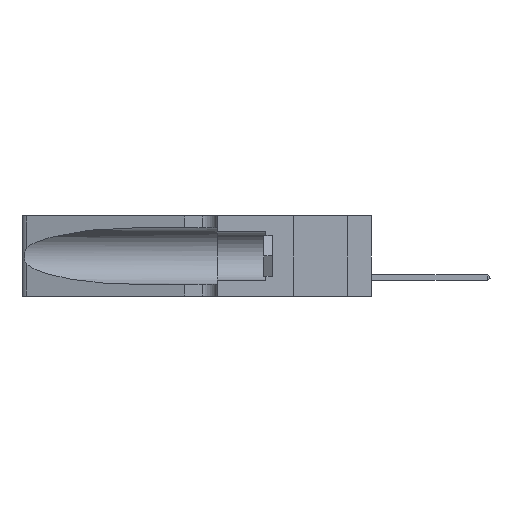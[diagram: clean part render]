
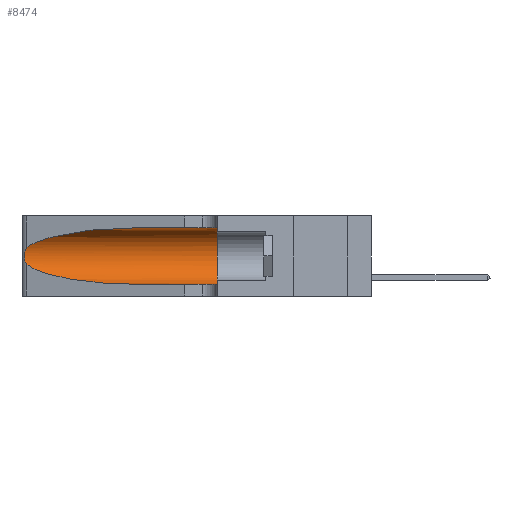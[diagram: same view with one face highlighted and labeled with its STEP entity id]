
A CAD part, left-side view. The second image highlights one B-rep face of the part: STEP entity #8474.
In plain terms, the highlighted cylindrical face has radius 3.308 mm (diameter 6.617 mm), a partial arc.
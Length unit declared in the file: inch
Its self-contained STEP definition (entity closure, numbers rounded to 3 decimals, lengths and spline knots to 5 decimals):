
#610 = VERTEX_POINT ( 'NONE', #5513 ) ;
#1059 = CARTESIAN_POINT ( 'NONE',  ( 0.25639, 1.23184, 0.21858 ) ) ;
#1222 = DIRECTION ( 'NONE',  ( 0., -1., 0. ) ) ;
#1430 = FACE_OUTER_BOUND ( 'NONE', #3080, .T. ) ;
#1438 =( BOUNDED_CURVE ( )  B_SPLINE_CURVE ( 3, ( #1781, #30792, #2269, #8991 ),
 .UNSPECIFIED., .F., .F. ) 
 B_SPLINE_CURVE_WITH_KNOTS ( ( 4, 4 ),
 ( 1.5708, 2.84003 ),
 .UNSPECIFIED. ) 
 CURVE ( )  GEOMETRIC_REPRESENTATION_ITEM ( )  RATIONAL_B_SPLINE_CURVE ( ( 1., 0.87, 0.87, 1. ) ) 
 REPRESENTATION_ITEM ( '' )  );
#1781 = CARTESIAN_POINT ( 'NONE',  ( 0.1305, 0.72297, 0.31525 ) ) ;
#1903 = CARTESIAN_POINT ( 'NONE',  ( 0.2373, 1.15595, 0.08982 ) ) ;
#2073 = CARTESIAN_POINT ( 'NONE',  ( 0.1305, 0.72297, 0.05475 ) ) ;
#2269 = CARTESIAN_POINT ( 'NONE',  ( 0.2373, 1.15595, 0.28018 ) ) ;
#2983 = CARTESIAN_POINT ( 'NONE',  ( 0.25789, 1.23486, 0.15765 ) ) ;
#3080 = EDGE_LOOP ( 'NONE', ( #33005, #5536, #32634, #36793, #13615, #35650 ) ) ;
#3566 = VERTEX_POINT ( 'NONE', #28455 ) ;
#5513 = CARTESIAN_POINT ( 'NONE',  ( 0.1305, 0.35, 0.05475 ) ) ;
#5536 = ORIENTED_EDGE ( 'NONE', *, *, #34141, .T. ) ;
#5541 = VECTOR ( 'NONE', #1222, 39.37008 ) ;
#5923 = CARTESIAN_POINT ( 'NONE',  ( 0.25787, 1.23484, 0.2124 ) ) ;
#6444 = DIRECTION ( 'NONE',  ( 0., 0., -1. ) ) ;
#7768 = CARTESIAN_POINT ( 'NONE',  ( 0.25856, 1.23593, 0.16098 ) ) ;
#8166 = CYLINDRICAL_SURFACE ( 'NONE', #24331, 0.13025 ) ;
#8474 = ADVANCED_FACE ( 'NONE', ( #1430 ), #8166, .F. ) ;
#8942 = EDGE_CURVE ( 'NONE', #27003, #3566, #13263, .T. ) ;
#8991 = CARTESIAN_POINT ( 'NONE',  ( 0.25487, 1.22718, 0.22369 ) ) ;
#10820 = EDGE_CURVE ( 'NONE', #31701, #45559, #1438, .T. ) ;
#13191 = CARTESIAN_POINT ( 'NONE',  ( 0.26075, 1.23896, 0.178 ) ) ;
#13263 =( BOUNDED_CURVE ( )  B_SPLINE_CURVE ( 3, ( #30753, #1903, #41565, #2073 ),
 .UNSPECIFIED., .F., .F. ) 
 B_SPLINE_CURVE_WITH_KNOTS ( ( 4, 4 ),
 ( 3.44316, 4.71239 ),
 .UNSPECIFIED. ) 
 CURVE ( )  GEOMETRIC_REPRESENTATION_ITEM ( )  RATIONAL_B_SPLINE_CURVE ( ( 1., 0.87, 0.87, 1. ) ) 
 REPRESENTATION_ITEM ( '' )  );
#13466 = EDGE_CURVE ( 'NONE', #35934, #610, #22303, .T. ) ;
#13615 = ORIENTED_EDGE ( 'NONE', *, *, #13466, .F. ) ;
#15055 = CARTESIAN_POINT ( 'NONE',  ( 0.25487, 1.22718, 0.14631 ) ) ;
#15162 = CARTESIAN_POINT ( 'NONE',  ( 0.25487, 1.22718, 0.22369 ) ) ;
#15332 = CARTESIAN_POINT ( 'NONE',  ( 0.1305, 1.61858, 0.31525 ) ) ;
#16100 = CARTESIAN_POINT ( 'NONE',  ( 0.26018, 1.23835, 0.19895 ) ) ;
#16700 = B_SPLINE_CURVE_WITH_KNOTS ( 'NONE', 3,
 ( #15162, #22535, #1059, #5923, #30365, #16100, #20369, #13191, #43720, #7768, #2983, #28661, #33685, #15055 ),
 .UNSPECIFIED., .F., .F.,
 ( 4, 2, 2, 2, 2, 2, 4 ),
 ( 0., 0.00027, 0.00053, 0.00107, 0.0016, 0.00187, 0.00214 ),
 .UNSPECIFIED. ) ;
#20023 = CARTESIAN_POINT ( 'NONE',  ( 0.1305, 1.61858, 0.05475 ) ) ;
#20369 = CARTESIAN_POINT ( 'NONE',  ( 0.26075, 1.23896, 0.19203 ) ) ;
#21052 = CARTESIAN_POINT ( 'NONE',  ( 0.1305, 0.35, 0.31525 ) ) ;
#22002 = DIRECTION ( 'NONE',  ( 0., 0., 1. ) ) ;
#22303 = CIRCLE ( 'NONE', #28878, 0.13025 ) ;
#22535 = CARTESIAN_POINT ( 'NONE',  ( 0.25555, 1.22994, 0.2215 ) ) ;
#24169 = DIRECTION ( 'NONE',  ( 0., -1., 0. ) ) ;
#24331 = AXIS2_PLACEMENT_3D ( 'NONE', #40623, #24169, #6444 ) ;
#24701 = CARTESIAN_POINT ( 'NONE',  ( 0.25487, 1.22718, 0.22369 ) ) ;
#26299 = LINE ( 'NONE', #15332, #5541 ) ;
#27003 = VERTEX_POINT ( 'NONE', #43177 ) ;
#27253 = VECTOR ( 'NONE', #45034, 39.37008 ) ;
#28416 = LINE ( 'NONE', #20023, #27253 ) ;
#28455 = CARTESIAN_POINT ( 'NONE',  ( 0.1305, 0.72297, 0.05475 ) ) ;
#28661 = CARTESIAN_POINT ( 'NONE',  ( 0.25639, 1.23186, 0.15144 ) ) ;
#28878 = AXIS2_PLACEMENT_3D ( 'NONE', #36019, #32661, #22002 ) ;
#30365 = CARTESIAN_POINT ( 'NONE',  ( 0.25854, 1.2359, 0.20912 ) ) ;
#30753 = CARTESIAN_POINT ( 'NONE',  ( 0.25487, 1.22718, 0.14631 ) ) ;
#30792 = CARTESIAN_POINT ( 'NONE',  ( 0.18966, 0.96281, 0.31525 ) ) ;
#31701 = VERTEX_POINT ( 'NONE', #33312 ) ;
#31839 = EDGE_CURVE ( 'NONE', #3566, #610, #28416, .T. ) ;
#32634 = ORIENTED_EDGE ( 'NONE', *, *, #8942, .T. ) ;
#32661 = DIRECTION ( 'NONE',  ( 0., 1., 0. ) ) ;
#33005 = ORIENTED_EDGE ( 'NONE', *, *, #10820, .T. ) ;
#33312 = CARTESIAN_POINT ( 'NONE',  ( 0.1305, 0.72297, 0.31525 ) ) ;
#33685 = CARTESIAN_POINT ( 'NONE',  ( 0.25555, 1.22993, 0.14849 ) ) ;
#34141 = EDGE_CURVE ( 'NONE', #45559, #27003, #16700, .T. ) ;
#35650 = ORIENTED_EDGE ( 'NONE', *, *, #43153, .F. ) ;
#35934 = VERTEX_POINT ( 'NONE', #21052 ) ;
#36019 = CARTESIAN_POINT ( 'NONE',  ( 0.1305, 0.35, 0.185 ) ) ;
#36793 = ORIENTED_EDGE ( 'NONE', *, *, #31839, .T. ) ;
#40623 = CARTESIAN_POINT ( 'NONE',  ( 0.1305, 1.61858, 0.185 ) ) ;
#41565 = CARTESIAN_POINT ( 'NONE',  ( 0.18966, 0.96281, 0.05475 ) ) ;
#43153 = EDGE_CURVE ( 'NONE', #31701, #35934, #26299, .T. ) ;
#43177 = CARTESIAN_POINT ( 'NONE',  ( 0.25487, 1.22718, 0.14631 ) ) ;
#43720 = CARTESIAN_POINT ( 'NONE',  ( 0.26017, 1.23833, 0.17102 ) ) ;
#45034 = DIRECTION ( 'NONE',  ( 0., -1., 0. ) ) ;
#45559 = VERTEX_POINT ( 'NONE', #24701 ) ;
